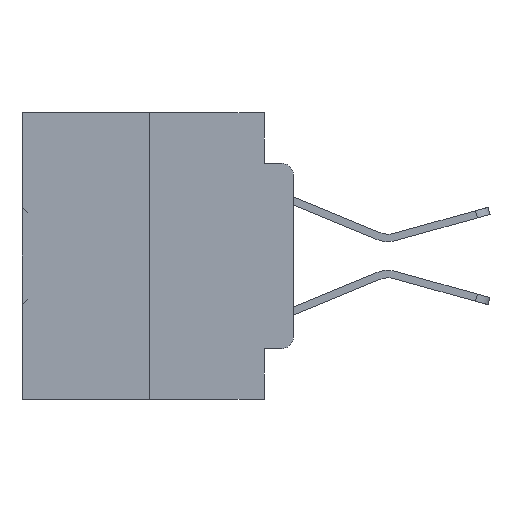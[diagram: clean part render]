
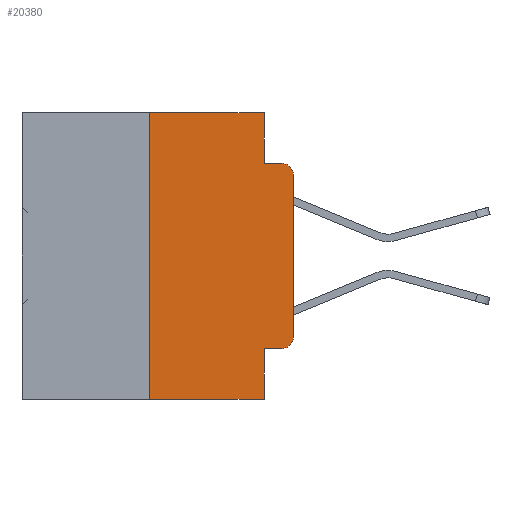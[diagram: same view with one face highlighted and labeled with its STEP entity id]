
A CAD part, left-side view. The second image highlights one B-rep face of the part: STEP entity #20380.
In plain terms, the highlighted planar face has unit normal (-1, 0, 0).
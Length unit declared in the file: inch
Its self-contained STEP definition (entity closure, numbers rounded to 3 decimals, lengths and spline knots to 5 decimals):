
#220 = ORIENTED_EDGE ( 'NONE', *, *, #17543, .T. ) ;
#248 = CARTESIAN_POINT ( 'NONE',  ( 0., 0.473, -0.5 ) ) ;
#1025 = PLANE ( 'NONE',  #21722 ) ;
#1126 = VECTOR ( 'NONE', #12083, 39.37008 ) ;
#1221 = CARTESIAN_POINT ( 'NONE',  ( 0., 0., -0.1085 ) ) ;
#1277 = CARTESIAN_POINT ( 'NONE',  ( 0., 0.051, -0.0885 ) ) ;
#1659 = EDGE_CURVE ( 'NONE', #34929, #4273, #8850, .T. ) ;
#3171 = CARTESIAN_POINT ( 'NONE',  ( 0., 0.051, -0.5 ) ) ;
#3266 = ORIENTED_EDGE ( 'NONE', *, *, #1659, .T. ) ;
#3749 = ORIENTED_EDGE ( 'NONE', *, *, #35558, .T. ) ;
#4239 = LINE ( 'NONE', #22150, #17449 ) ;
#4273 = VERTEX_POINT ( 'NONE', #3171 ) ;
#4658 = DIRECTION ( 'NONE',  ( 0., -1., 0. ) ) ;
#5079 = VERTEX_POINT ( 'NONE', #1277 ) ;
#5932 = CARTESIAN_POINT ( 'NONE',  ( 0., 0.25, 0. ) ) ;
#6309 = VERTEX_POINT ( 'NONE', #15966 ) ;
#6403 = CARTESIAN_POINT ( 'NONE',  ( 0., 0., -0.3915 ) ) ;
#6488 = VERTEX_POINT ( 'NONE', #19306 ) ;
#6915 = ORIENTED_EDGE ( 'NONE', *, *, #22333, .F. ) ;
#7516 = CARTESIAN_POINT ( 'NONE',  ( 0., 0., 0. ) ) ;
#7569 = VERTEX_POINT ( 'NONE', #1221 ) ;
#7705 = CARTESIAN_POINT ( 'NONE',  ( 0., 0.25, 0. ) ) ;
#7834 = VECTOR ( 'NONE', #30278, 39.37008 ) ;
#8135 = FACE_OUTER_BOUND ( 'NONE', #25774, .T. ) ;
#8850 = LINE ( 'NONE', #248, #1126 ) ;
#8914 = ORIENTED_EDGE ( 'NONE', *, *, #32534, .F. ) ;
#10101 = LINE ( 'NONE', #15162, #7834 ) ;
#10275 = CARTESIAN_POINT ( 'NONE',  ( 0., 0.473, 0. ) ) ;
#11530 = CARTESIAN_POINT ( 'NONE',  ( 0., 0.051, -0.0885 ) ) ;
#12055 = VECTOR ( 'NONE', #30969, 39.37008 ) ;
#12083 = DIRECTION ( 'NONE',  ( 0., -1., 0. ) ) ;
#12357 = VERTEX_POINT ( 'NONE', #33858 ) ;
#14770 = CARTESIAN_POINT ( 'NONE',  ( 0., 0.02, -0.3915 ) ) ;
#15162 = CARTESIAN_POINT ( 'NONE',  ( 0., 0.051, 0. ) ) ;
#15328 = AXIS2_PLACEMENT_3D ( 'NONE', #14770, #34878, #32197 ) ;
#15966 = CARTESIAN_POINT ( 'NONE',  ( 0., 0.051, 0. ) ) ;
#16103 = CARTESIAN_POINT ( 'NONE',  ( 0., 0.051, 0. ) ) ;
#17109 = VERTEX_POINT ( 'NONE', #7705 ) ;
#17130 = DIRECTION ( 'NONE',  ( 0., -1., 0. ) ) ;
#17449 = VECTOR ( 'NONE', #4658, 39.37008 ) ;
#17543 = EDGE_CURVE ( 'NONE', #6488, #26575, #4239, .T. ) ;
#18654 = EDGE_CURVE ( 'NONE', #6309, #5079, #10101, .T. ) ;
#19306 = CARTESIAN_POINT ( 'NONE',  ( 0., 0.051, -0.4115 ) ) ;
#19695 = LINE ( 'NONE', #16103, #23382 ) ;
#20380 = ADVANCED_FACE ( 'NONE', ( #8135 ), #1025, .F. ) ;
#20412 = LINE ( 'NONE', #10275, #33225 ) ;
#20647 = EDGE_CURVE ( 'NONE', #7569, #12357, #20949, .T. ) ;
#20949 = CIRCLE ( 'NONE', #36196, 0.02 ) ;
#21495 = CARTESIAN_POINT ( 'NONE',  ( 0., 0.02, -0.4115 ) ) ;
#21722 = AXIS2_PLACEMENT_3D ( 'NONE', #33097, #36171, #24779 ) ;
#22150 = CARTESIAN_POINT ( 'NONE',  ( 0., 0.051, -0.4115 ) ) ;
#22333 = EDGE_CURVE ( 'NONE', #6488, #4273, #19695, .T. ) ;
#23382 = VECTOR ( 'NONE', #30487, 39.37008 ) ;
#24423 = ORIENTED_EDGE ( 'NONE', *, *, #33443, .F. ) ;
#24730 = CIRCLE ( 'NONE', #15328, 0.02 ) ;
#24779 = DIRECTION ( 'NONE',  ( 0., 0., -1. ) ) ;
#25774 = EDGE_LOOP ( 'NONE', ( #32751, #31360, #33796, #32900, #8914, #24423, #3266, #6915, #220, #3749 ) ) ;
#26280 = DIRECTION ( 'NONE',  ( 0., 0., 1. ) ) ;
#26333 = LINE ( 'NONE', #5932, #34555 ) ;
#26391 = CARTESIAN_POINT ( 'NONE',  ( 0., 0.25, -0.5 ) ) ;
#26575 = VERTEX_POINT ( 'NONE', #21495 ) ;
#27244 = VERTEX_POINT ( 'NONE', #6403 ) ;
#28346 = DIRECTION ( 'NONE',  ( 0., -1., 0. ) ) ;
#28884 = CARTESIAN_POINT ( 'NONE',  ( 0., 0.02, -0.1085 ) ) ;
#29513 = LINE ( 'NONE', #7516, #12055 ) ;
#30278 = DIRECTION ( 'NONE',  ( 0., 0., -1. ) ) ;
#30487 = DIRECTION ( 'NONE',  ( 0., 0., -1. ) ) ;
#30600 = VECTOR ( 'NONE', #17130, 39.37008 ) ;
#30654 = EDGE_CURVE ( 'NONE', #5079, #12357, #36080, .T. ) ;
#30969 = DIRECTION ( 'NONE',  ( 0., 0., 1. ) ) ;
#31360 = ORIENTED_EDGE ( 'NONE', *, *, #20647, .T. ) ;
#32197 = DIRECTION ( 'NONE',  ( 0., 0., -1. ) ) ;
#32534 = EDGE_CURVE ( 'NONE', #17109, #6309, #20412, .T. ) ;
#32751 = ORIENTED_EDGE ( 'NONE', *, *, #33735, .T. ) ;
#32900 = ORIENTED_EDGE ( 'NONE', *, *, #18654, .F. ) ;
#33097 = CARTESIAN_POINT ( 'NONE',  ( 0., 0.473, 0. ) ) ;
#33225 = VECTOR ( 'NONE', #28346, 39.37008 ) ;
#33443 = EDGE_CURVE ( 'NONE', #34929, #17109, #26333, .T. ) ;
#33735 = EDGE_CURVE ( 'NONE', #27244, #7569, #29513, .T. ) ;
#33796 = ORIENTED_EDGE ( 'NONE', *, *, #30654, .F. ) ;
#33858 = CARTESIAN_POINT ( 'NONE',  ( 0., 0.02, -0.0885 ) ) ;
#34555 = VECTOR ( 'NONE', #26280, 39.37008 ) ;
#34878 = DIRECTION ( 'NONE',  ( -1., 0., 0. ) ) ;
#34929 = VERTEX_POINT ( 'NONE', #26391 ) ;
#35558 = EDGE_CURVE ( 'NONE', #26575, #27244, #24730, .T. ) ;
#36080 = LINE ( 'NONE', #11530, #30600 ) ;
#36171 = DIRECTION ( 'NONE',  ( 1., 0., 0. ) ) ;
#36196 = AXIS2_PLACEMENT_3D ( 'NONE', #28884, #37694, #37192 ) ;
#37192 = DIRECTION ( 'NONE',  ( 0., 0., -1. ) ) ;
#37694 = DIRECTION ( 'NONE',  ( -1., 0., 0. ) ) ;
